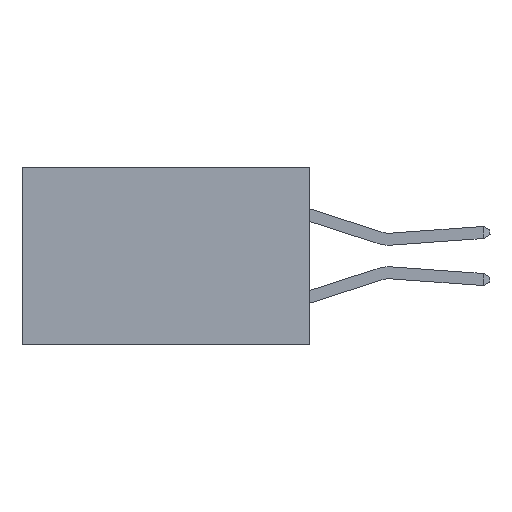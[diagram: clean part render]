
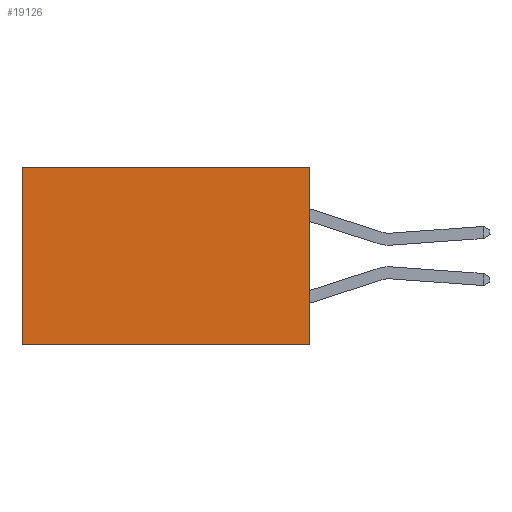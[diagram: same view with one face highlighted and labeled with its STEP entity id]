
A CAD part, left-side view. The second image highlights one B-rep face of the part: STEP entity #19126.
In plain terms, the highlighted planar face has unit normal (-1, 0, 0).
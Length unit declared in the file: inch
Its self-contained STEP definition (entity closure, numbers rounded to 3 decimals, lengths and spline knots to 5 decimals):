
#1644 = CARTESIAN_POINT ( 'NONE',  ( 0.298, 0., 0. ) ) ;
#4614 = VECTOR ( 'NONE', #16483, 39.37008 ) ;
#5840 = EDGE_CURVE ( 'NONE', #8636, #23496, #15625, .T. ) ;
#6055 = LINE ( 'NONE', #27892, #4614 ) ;
#8160 = CARTESIAN_POINT ( 'NONE',  ( 0.298, 0.6, 0. ) ) ;
#8636 = VERTEX_POINT ( 'NONE', #25166 ) ;
#8685 = DIRECTION ( 'NONE',  ( 1., 0., 0. ) ) ;
#9604 = VECTOR ( 'NONE', #15127, 39.37008 ) ;
#9851 = CARTESIAN_POINT ( 'NONE',  ( 0.298, 0., -0.37 ) ) ;
#10047 = CARTESIAN_POINT ( 'NONE',  ( 0.298, 0.6, -0.37 ) ) ;
#10126 = DIRECTION ( 'NONE',  ( 0., 1., 0. ) ) ;
#13873 = ORIENTED_EDGE ( 'NONE', *, *, #5840, .T. ) ;
#13898 = EDGE_CURVE ( 'NONE', #23496, #18273, #16413, .T. ) ;
#14048 = VERTEX_POINT ( 'NONE', #18244 ) ;
#14469 = DIRECTION ( 'NONE',  ( 0., 1., 0. ) ) ;
#15127 = DIRECTION ( 'NONE',  ( 0., 0., -1. ) ) ;
#15625 = LINE ( 'NONE', #23865, #28518 ) ;
#16413 = LINE ( 'NONE', #8160, #9604 ) ;
#16483 = DIRECTION ( 'NONE',  ( 0., 0., -1. ) ) ;
#17493 = VECTOR ( 'NONE', #14469, 39.37008 ) ;
#18117 = EDGE_CURVE ( 'NONE', #8636, #14048, #6055, .T. ) ;
#18244 = CARTESIAN_POINT ( 'NONE',  ( 0.298, 0., -0.37 ) ) ;
#18273 = VERTEX_POINT ( 'NONE', #10047 ) ;
#18726 = ORIENTED_EDGE ( 'NONE', *, *, #28836, .F. ) ;
#19126 = ADVANCED_FACE ( 'NONE', ( #26549 ), #22437, .F. ) ;
#20561 = CARTESIAN_POINT ( 'NONE',  ( 0.298, 0.6, 0. ) ) ;
#22437 = PLANE ( 'NONE',  #26856 ) ;
#23496 = VERTEX_POINT ( 'NONE', #20561 ) ;
#23604 = LINE ( 'NONE', #9851, #17493 ) ;
#23865 = CARTESIAN_POINT ( 'NONE',  ( 0.298, 0., 0. ) ) ;
#23908 = EDGE_LOOP ( 'NONE', ( #28617, #18726, #25143, #13873 ) ) ;
#24756 = DIRECTION ( 'NONE',  ( 0., 0., -1. ) ) ;
#25143 = ORIENTED_EDGE ( 'NONE', *, *, #18117, .F. ) ;
#25166 = CARTESIAN_POINT ( 'NONE',  ( 0.298, 0., 0. ) ) ;
#26549 = FACE_OUTER_BOUND ( 'NONE', #23908, .T. ) ;
#26856 = AXIS2_PLACEMENT_3D ( 'NONE', #1644, #8685, #24756 ) ;
#27892 = CARTESIAN_POINT ( 'NONE',  ( 0.298, 0., 0. ) ) ;
#28518 = VECTOR ( 'NONE', #10126, 39.37008 ) ;
#28617 = ORIENTED_EDGE ( 'NONE', *, *, #13898, .T. ) ;
#28836 = EDGE_CURVE ( 'NONE', #14048, #18273, #23604, .T. ) ;
